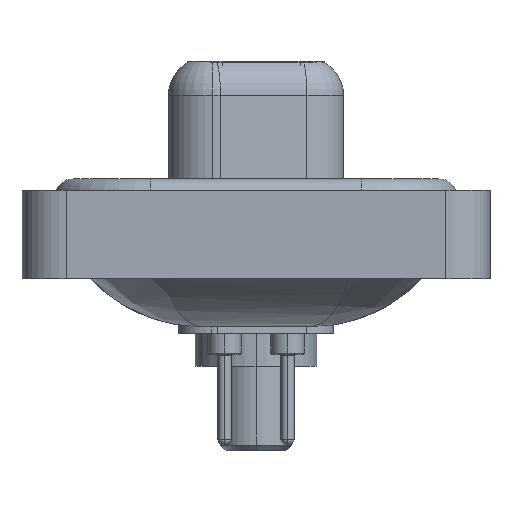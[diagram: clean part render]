
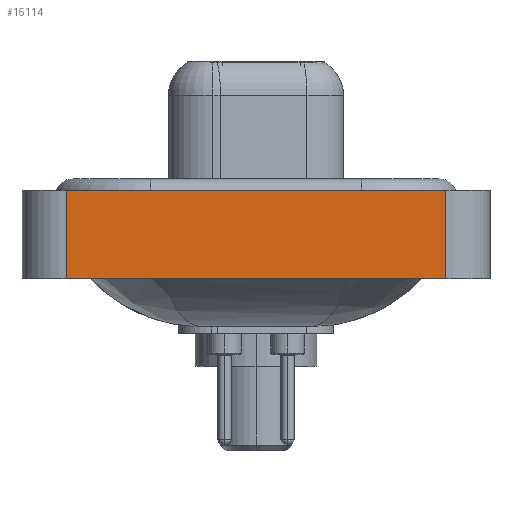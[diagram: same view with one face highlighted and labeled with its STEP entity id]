
A CAD part, left-side view. The second image highlights one B-rep face of the part: STEP entity #15114.
In plain terms, the highlighted planar face has unit normal (-1, 0, 0).
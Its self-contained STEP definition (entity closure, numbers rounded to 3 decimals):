
#40 = VERTEX_POINT ( 'NONE', #13389 ) ;
#237 = LINE ( 'NONE', #18258, #14595 ) ;
#560 = EDGE_CURVE ( 'NONE', #1618, #9692, #19378, .T. ) ;
#564 = CARTESIAN_POINT ( 'NONE',  ( -7.25, -8.55, 0.4 ) ) ;
#1298 = VECTOR ( 'NONE', #13267, 1000. ) ;
#1618 = VERTEX_POINT ( 'NONE', #9072 ) ;
#1668 = EDGE_LOOP ( 'NONE', ( #7944, #7678, #14712, #19134 ) ) ;
#2332 = VECTOR ( 'NONE', #17264, 1000. ) ;
#2403 = CARTESIAN_POINT ( 'NONE',  ( -7.25, -8.55, -3.6 ) ) ;
#2581 = PLANE ( 'NONE',  #7547 ) ;
#3726 = LINE ( 'NONE', #564, #2332 ) ;
#4113 = DIRECTION ( 'NONE',  ( 0., 0., 1. ) ) ;
#5112 = EDGE_CURVE ( 'NONE', #9692, #7503, #14420, .T. ) ;
#6412 = EDGE_CURVE ( 'NONE', #40, #7503, #3726, .T. ) ;
#6427 = CARTESIAN_POINT ( 'NONE',  ( -7.25, -8.55, 0.4 ) ) ;
#6859 = VECTOR ( 'NONE', #9921, 1000. ) ;
#7503 = VERTEX_POINT ( 'NONE', #6427 ) ;
#7547 = AXIS2_PLACEMENT_3D ( 'NONE', #13257, #17773, #4113 ) ;
#7678 = ORIENTED_EDGE ( 'NONE', *, *, #6412, .F. ) ;
#7944 = ORIENTED_EDGE ( 'NONE', *, *, #5112, .T. ) ;
#9072 = CARTESIAN_POINT ( 'NONE',  ( -7.25, 8.55, -3.6 ) ) ;
#9692 = VERTEX_POINT ( 'NONE', #10892 ) ;
#9921 = DIRECTION ( 'NONE',  ( 0., 0., 1. ) ) ;
#10114 = CARTESIAN_POINT ( 'NONE',  ( -7.25, -8.55, -3.6 ) ) ;
#10892 = CARTESIAN_POINT ( 'NONE',  ( -7.25, -8.55, -3.6 ) ) ;
#13257 = CARTESIAN_POINT ( 'NONE',  ( -7.25, -8.55, -3.6 ) ) ;
#13267 = DIRECTION ( 'NONE',  ( 0., -1., 0. ) ) ;
#13389 = CARTESIAN_POINT ( 'NONE',  ( -7.25, 8.55, 0.4 ) ) ;
#13449 = FACE_OUTER_BOUND ( 'NONE', #1668, .T. ) ;
#14420 = LINE ( 'NONE', #10114, #6859 ) ;
#14595 = VECTOR ( 'NONE', #18352, 1000. ) ;
#14712 = ORIENTED_EDGE ( 'NONE', *, *, #15314, .F. ) ;
#15114 = ADVANCED_FACE ( 'NONE', ( #13449 ), #2581, .T. ) ;
#15314 = EDGE_CURVE ( 'NONE', #1618, #40, #237, .T. ) ;
#17264 = DIRECTION ( 'NONE',  ( 0., -1., 0. ) ) ;
#17773 = DIRECTION ( 'NONE',  ( -1., 0., 0. ) ) ;
#18258 = CARTESIAN_POINT ( 'NONE',  ( -7.25, 8.55, -3.6 ) ) ;
#18352 = DIRECTION ( 'NONE',  ( 0., 0., 1. ) ) ;
#19134 = ORIENTED_EDGE ( 'NONE', *, *, #560, .T. ) ;
#19378 = LINE ( 'NONE', #2403, #1298 ) ;
